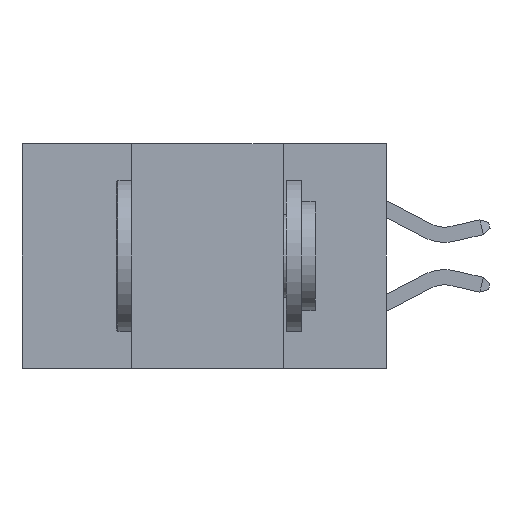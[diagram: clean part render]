
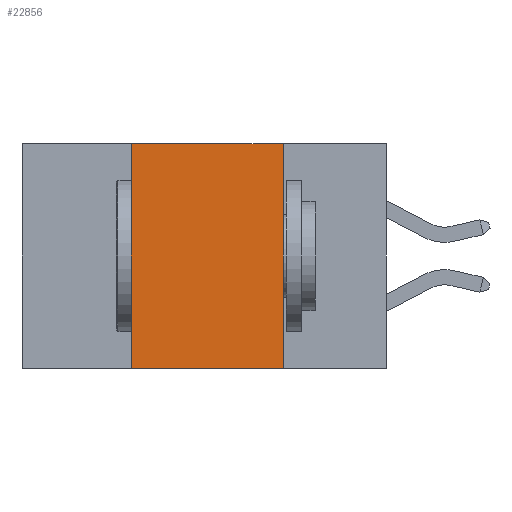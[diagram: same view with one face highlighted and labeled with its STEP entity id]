
A CAD part, left-side view. The second image highlights one B-rep face of the part: STEP entity #22856.
In plain terms, the highlighted planar face has unit normal (-1, 0, 0).
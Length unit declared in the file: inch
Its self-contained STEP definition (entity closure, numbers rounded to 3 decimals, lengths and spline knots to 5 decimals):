
#1218 = LINE ( 'NONE', #8654, #10276 ) ;
#2306 = VECTOR ( 'NONE', #7472, 39.37008 ) ;
#2870 = ORIENTED_EDGE ( 'NONE', *, *, #21715, .F. ) ;
#3499 = CARTESIAN_POINT ( 'NONE',  ( 0., 0.6, 0. ) ) ;
#3674 = AXIS2_PLACEMENT_3D ( 'NONE', #3499, #8955, #21476 ) ;
#4059 = CARTESIAN_POINT ( 'NONE',  ( 0., 0.42, 0. ) ) ;
#4614 = EDGE_LOOP ( 'NONE', ( #16042, #20854, #2870, #12447 ) ) ;
#5437 = CARTESIAN_POINT ( 'NONE',  ( 0., 0.17, 0. ) ) ;
#5643 = CARTESIAN_POINT ( 'NONE',  ( 0., 0.42, 0. ) ) ;
#7106 = LINE ( 'NONE', #5643, #2306 ) ;
#7167 = VERTEX_POINT ( 'NONE', #4059 ) ;
#7432 = EDGE_CURVE ( 'NONE', #9412, #16186, #22022, .T. ) ;
#7472 = DIRECTION ( 'NONE',  ( 0., 0., 1. ) ) ;
#8000 = EDGE_CURVE ( 'NONE', #7167, #9412, #1218, .T. ) ;
#8500 = LINE ( 'NONE', #12775, #22211 ) ;
#8654 = CARTESIAN_POINT ( 'NONE',  ( 0., 0.6, 0. ) ) ;
#8955 = DIRECTION ( 'NONE',  ( 1., 0., 0. ) ) ;
#9412 = VERTEX_POINT ( 'NONE', #5437 ) ;
#9801 = VERTEX_POINT ( 'NONE', #17004 ) ;
#10276 = VECTOR ( 'NONE', #16535, 39.37008 ) ;
#11560 = CARTESIAN_POINT ( 'NONE',  ( 0., 0.17, -0.37 ) ) ;
#12447 = ORIENTED_EDGE ( 'NONE', *, *, #14937, .T. ) ;
#12775 = CARTESIAN_POINT ( 'NONE',  ( 0., 0.6, -0.37 ) ) ;
#14556 = DIRECTION ( 'NONE',  ( 0., -1., 0. ) ) ;
#14937 = EDGE_CURVE ( 'NONE', #9801, #16186, #8500, .T. ) ;
#15563 = DIRECTION ( 'NONE',  ( 0., 0., -1. ) ) ;
#16025 = PLANE ( 'NONE',  #3674 ) ;
#16042 = ORIENTED_EDGE ( 'NONE', *, *, #7432, .F. ) ;
#16186 = VERTEX_POINT ( 'NONE', #11560 ) ;
#16535 = DIRECTION ( 'NONE',  ( 0., -1., 0. ) ) ;
#17004 = CARTESIAN_POINT ( 'NONE',  ( 0., 0.42, -0.37 ) ) ;
#17261 = VECTOR ( 'NONE', #15563, 39.37008 ) ;
#20531 = FACE_OUTER_BOUND ( 'NONE', #4614, .T. ) ;
#20854 = ORIENTED_EDGE ( 'NONE', *, *, #8000, .F. ) ;
#21476 = DIRECTION ( 'NONE',  ( 0., 0., -1. ) ) ;
#21715 = EDGE_CURVE ( 'NONE', #9801, #7167, #7106, .T. ) ;
#22022 = LINE ( 'NONE', #22129, #17261 ) ;
#22129 = CARTESIAN_POINT ( 'NONE',  ( 0., 0.17, 0. ) ) ;
#22211 = VECTOR ( 'NONE', #14556, 39.37008 ) ;
#22856 = ADVANCED_FACE ( 'NONE', ( #20531 ), #16025, .F. ) ;
